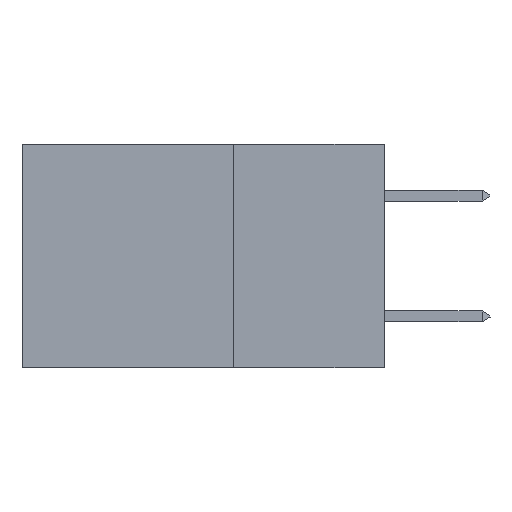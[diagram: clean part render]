
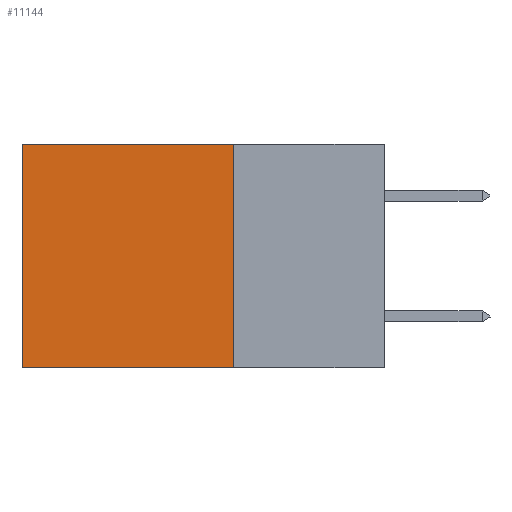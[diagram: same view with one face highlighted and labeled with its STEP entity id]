
A CAD part, left-side view. The second image highlights one B-rep face of the part: STEP entity #11144.
In plain terms, the highlighted planar face has unit normal (-1, 0, 0).
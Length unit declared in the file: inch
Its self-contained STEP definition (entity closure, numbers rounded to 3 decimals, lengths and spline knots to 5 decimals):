
#1719 = DIRECTION ( 'NONE',  ( 0., 0., -1. ) ) ;
#2161 = LINE ( 'NONE', #13328, #17180 ) ;
#3931 = DIRECTION ( 'NONE',  ( 0., 1., 0. ) ) ;
#4652 = DIRECTION ( 'NONE',  ( 0., 0., -1. ) ) ;
#5800 = FACE_OUTER_BOUND ( 'NONE', #23227, .T. ) ;
#7279 = DIRECTION ( 'NONE',  ( 0., 0., -1. ) ) ;
#7710 = ORIENTED_EDGE ( 'NONE', *, *, #38253, .T. ) ;
#8532 = VECTOR ( 'NONE', #7279, 39.37008 ) ;
#9847 = EDGE_CURVE ( 'NONE', #26776, #28902, #2161, .T. ) ;
#10391 = CARTESIAN_POINT ( 'NONE',  ( 0.2875, 0.6, 0. ) ) ;
#10663 = CARTESIAN_POINT ( 'NONE',  ( 0.2875, 0.25, 0. ) ) ;
#11144 = ADVANCED_FACE ( 'NONE', ( #5800 ), #13525, .F. ) ;
#11677 = ORIENTED_EDGE ( 'NONE', *, *, #22226, .F. ) ;
#11903 = VERTEX_POINT ( 'NONE', #14715 ) ;
#13328 = CARTESIAN_POINT ( 'NONE',  ( 0.2875, 0.25, 0. ) ) ;
#13525 = PLANE ( 'NONE',  #26740 ) ;
#14715 = CARTESIAN_POINT ( 'NONE',  ( 0.2875, 0.25, -0.37 ) ) ;
#16957 = CARTESIAN_POINT ( 'NONE',  ( 0.2875, 0.25, 0. ) ) ;
#17180 = VECTOR ( 'NONE', #37395, 39.37008 ) ;
#18322 = EDGE_CURVE ( 'NONE', #11903, #29482, #36854, .T. ) ;
#19012 = CARTESIAN_POINT ( 'NONE',  ( 0.2875, 0.25, -0.37 ) ) ;
#22226 = EDGE_CURVE ( 'NONE', #26776, #11903, #24799, .T. ) ;
#23227 = EDGE_LOOP ( 'NONE', ( #7710, #27930, #11677, #25063 ) ) ;
#23848 = VECTOR ( 'NONE', #4652, 39.37008 ) ;
#24799 = LINE ( 'NONE', #16957, #23848 ) ;
#25063 = ORIENTED_EDGE ( 'NONE', *, *, #9847, .T. ) ;
#25651 = CARTESIAN_POINT ( 'NONE',  ( 0.2875, 0.6, 0. ) ) ;
#26740 = AXIS2_PLACEMENT_3D ( 'NONE', #10663, #28624, #1719 ) ;
#26776 = VERTEX_POINT ( 'NONE', #30465 ) ;
#27930 = ORIENTED_EDGE ( 'NONE', *, *, #18322, .F. ) ;
#28624 = DIRECTION ( 'NONE',  ( 1., 0., 0. ) ) ;
#28902 = VERTEX_POINT ( 'NONE', #10391 ) ;
#29482 = VERTEX_POINT ( 'NONE', #31068 ) ;
#30465 = CARTESIAN_POINT ( 'NONE',  ( 0.2875, 0.25, 0. ) ) ;
#31068 = CARTESIAN_POINT ( 'NONE',  ( 0.2875, 0.6, -0.37 ) ) ;
#36402 = VECTOR ( 'NONE', #3931, 39.37008 ) ;
#36731 = LINE ( 'NONE', #25651, #8532 ) ;
#36854 = LINE ( 'NONE', #19012, #36402 ) ;
#37395 = DIRECTION ( 'NONE',  ( 0., 1., 0. ) ) ;
#38253 = EDGE_CURVE ( 'NONE', #28902, #29482, #36731, .T. ) ;
